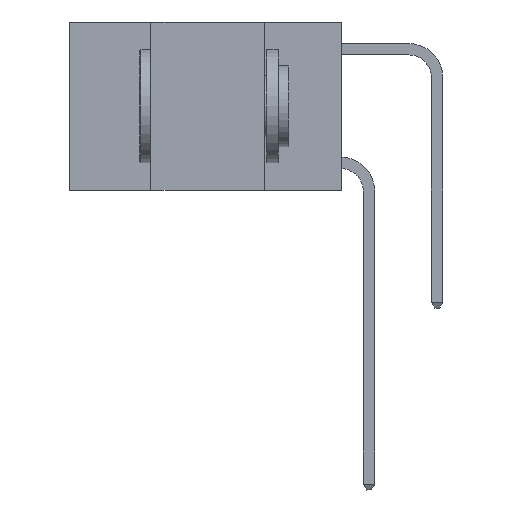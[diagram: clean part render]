
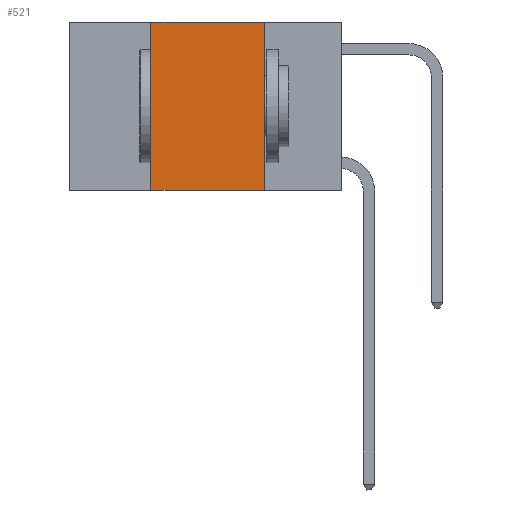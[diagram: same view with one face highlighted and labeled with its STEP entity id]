
A CAD part, left-side view. The second image highlights one B-rep face of the part: STEP entity #521.
In plain terms, the highlighted planar face has unit normal (-1, 0, 0).
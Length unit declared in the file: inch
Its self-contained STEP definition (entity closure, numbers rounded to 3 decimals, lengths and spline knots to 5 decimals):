
#94 = VECTOR ( 'NONE', #1090, 39.37008 ) ;
#327 = DIRECTION ( 'NONE',  ( 0., 0., -1. ) ) ;
#521 = ADVANCED_FACE ( 'NONE', ( #5713 ), #11297, .F. ) ;
#633 = AXIS2_PLACEMENT_3D ( 'NONE', #12445, #13401, #10116 ) ;
#1090 = DIRECTION ( 'NONE',  ( 0., 0., 1. ) ) ;
#1439 = ORIENTED_EDGE ( 'NONE', *, *, #9780, .F. ) ;
#1739 = ORIENTED_EDGE ( 'NONE', *, *, #13767, .T. ) ;
#2222 = VERTEX_POINT ( 'NONE', #5204 ) ;
#4771 = ORIENTED_EDGE ( 'NONE', *, *, #5480, .F. ) ;
#4791 = VERTEX_POINT ( 'NONE', #9788 ) ;
#5204 = CARTESIAN_POINT ( 'NONE',  ( 0., 0.42, 0. ) ) ;
#5480 = EDGE_CURVE ( 'NONE', #8140, #9148, #8718, .T. ) ;
#5569 = LINE ( 'NONE', #6600, #10655 ) ;
#5713 = FACE_OUTER_BOUND ( 'NONE', #9520, .T. ) ;
#5980 = CARTESIAN_POINT ( 'NONE',  ( 0., 0.17, 0. ) ) ;
#6587 = LINE ( 'NONE', #9953, #94 ) ;
#6600 = CARTESIAN_POINT ( 'NONE',  ( 0., 0.6, -0.37 ) ) ;
#7546 = LINE ( 'NONE', #11936, #11027 ) ;
#7754 = DIRECTION ( 'NONE',  ( 0., -1., 0. ) ) ;
#8140 = VERTEX_POINT ( 'NONE', #11814 ) ;
#8364 = ORIENTED_EDGE ( 'NONE', *, *, #11711, .F. ) ;
#8718 = LINE ( 'NONE', #5980, #12403 ) ;
#9148 = VERTEX_POINT ( 'NONE', #9361 ) ;
#9361 = CARTESIAN_POINT ( 'NONE',  ( 0., 0.17, -0.37 ) ) ;
#9520 = EDGE_LOOP ( 'NONE', ( #4771, #8364, #1439, #1739 ) ) ;
#9780 = EDGE_CURVE ( 'NONE', #4791, #2222, #6587, .T. ) ;
#9788 = CARTESIAN_POINT ( 'NONE',  ( 0., 0.42, -0.37 ) ) ;
#9953 = CARTESIAN_POINT ( 'NONE',  ( 0., 0.42, 0. ) ) ;
#10116 = DIRECTION ( 'NONE',  ( 0., 0., -1. ) ) ;
#10655 = VECTOR ( 'NONE', #7754, 39.37008 ) ;
#11027 = VECTOR ( 'NONE', #12007, 39.37008 ) ;
#11297 = PLANE ( 'NONE',  #633 ) ;
#11711 = EDGE_CURVE ( 'NONE', #2222, #8140, #7546, .T. ) ;
#11814 = CARTESIAN_POINT ( 'NONE',  ( 0., 0.17, 0. ) ) ;
#11936 = CARTESIAN_POINT ( 'NONE',  ( 0., 0.6, 0. ) ) ;
#12007 = DIRECTION ( 'NONE',  ( 0., -1., 0. ) ) ;
#12403 = VECTOR ( 'NONE', #327, 39.37008 ) ;
#12445 = CARTESIAN_POINT ( 'NONE',  ( 0., 0.6, 0. ) ) ;
#13401 = DIRECTION ( 'NONE',  ( 1., 0., 0. ) ) ;
#13767 = EDGE_CURVE ( 'NONE', #4791, #9148, #5569, .T. ) ;
